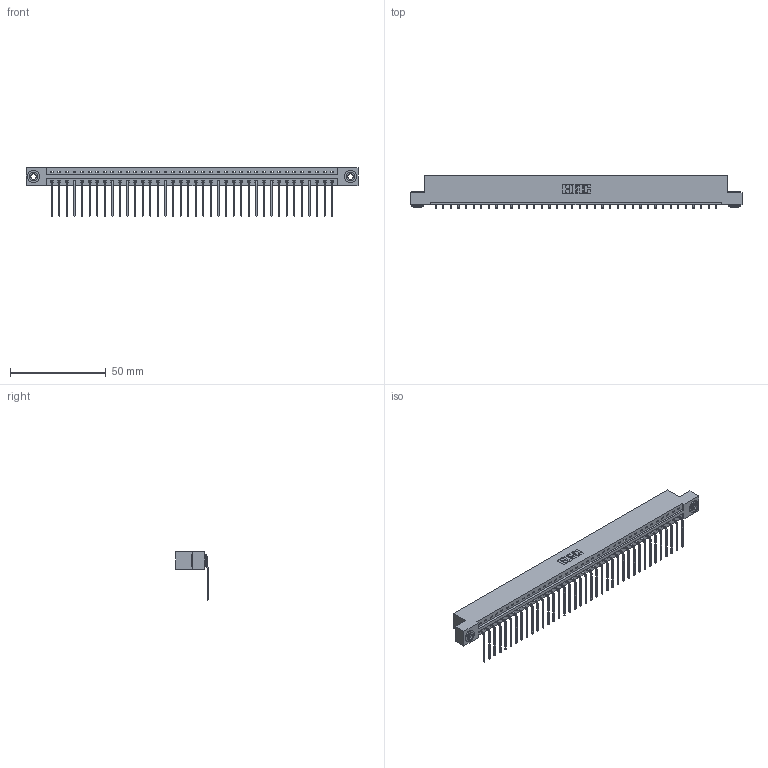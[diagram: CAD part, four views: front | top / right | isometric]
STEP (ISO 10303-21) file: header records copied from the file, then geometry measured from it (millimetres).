
FILE_DESCRIPTION (( 'STEP AP203' ), '1' );
FILE_NAME ('837-038-559-103.STEP', '2021-08-04T15:46:05', ( '' ), ( '' ), 'SwSTEP 2.0', 'SolidWorks 2020', '' );
FILE_SCHEMA (( 'CONFIG_CONTROL_DESIGN' ));
Length unit declared in the file: inch
Products named in the file (4): 837-038-559-103; 345-292-001_558 559 Tail - 1; 837 Part_Flush Mounting Lugs - 0.156 Dia-TH; 345-250-002_345-250-002-102
Assembly tree (41 placements, depth 2):
  837-038-559-103
    837 Part_Flush Mounting Lugs - 0.156 Dia-TH
    345-292-001_558 559 Tail - 1  x38
    345-250-002_345-250-002-102  x2
Bounding box: 173.58 x 17.09 x 25.53 mm (x, y, z)
Volume: 18137 mm3; surface area: 19730.3 mm2
Topology: 41 solids, 41 shells, 2584 faces, 7759 edges, 5118 vertices
Faces by surface type: plane 1904, cylinder 672, cone 8
Entity records: 29498 total; most frequent: CARTESIAN_POINT 5115, ORIENTED_EDGE 5082, DIRECTION 4347, EDGE_CURVE 2541, LINE 2389, VECTOR 2389, VERTEX_POINT 1690, AXIS2_PLACEMENT_3D 979
